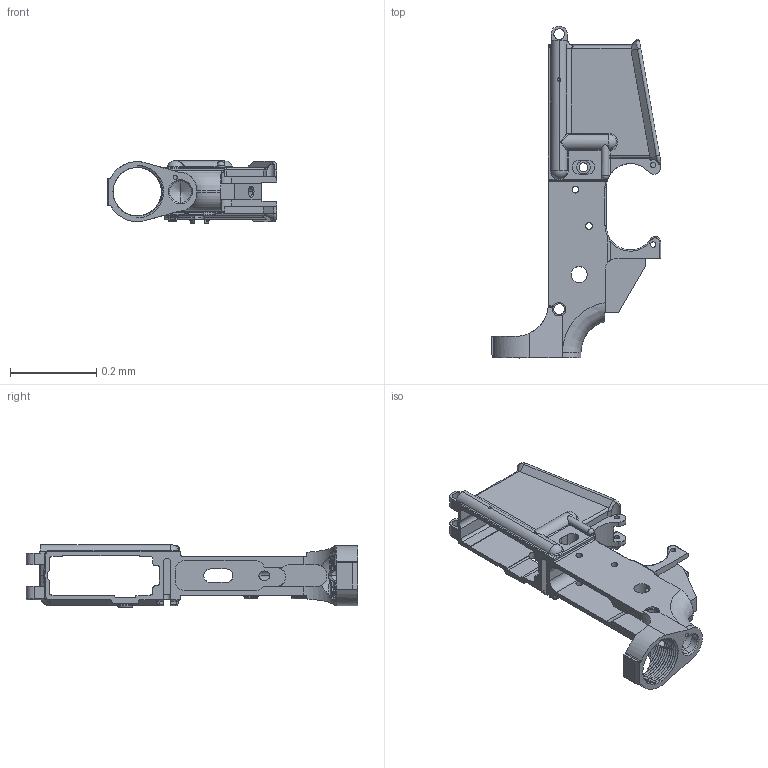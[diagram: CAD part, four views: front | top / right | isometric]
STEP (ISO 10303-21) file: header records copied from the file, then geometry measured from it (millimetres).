
FILE_DESCRIPTION(('CAx-IF Rec.Pracs.---Model Styling and Organization---1.2---2011-12-15','CAx-IF Rec.Pracs.---Geometric and Assembly Validation Properties---4.1---2014-06-16','CAx-IF Rec.Pracs.---PMI Polyline Presentation---2.0---2013-05-24'),'2;1');
FILE_NAME('AR15-lower-receiver-scale.stp','2017-10-16T01:32:52+08:00',('HyperWorksVersion-14.0.0.88'),(''),'STEP Interface 4.0 Sp3 by CT CoreTechnologie','3D_Kernel_IO4.0 Sp3 by CT CoreTechnologie','');
FILE_SCHEMA(('AUTOMOTIVE_DESIGN { 1 0 10303 214 1 1 1 1 }'));
Length unit declared in the file: millimetre
Products named in the file (1): AR15-lower-receiver-scale
Bounding box: 0.39 x 0.77 x 0.14 mm (x, y, z)
Surface area: 0.8 mm2 (no closed solid volume)
Topology: 0 solids, 2 shells, 511 faces, 1426 edges, 903 vertices
Faces by surface type: cylinder 234, plane 164, bspline 79, torus 28, sphere 6
Entity records: 40165 total; most frequent: CARTESIAN_POINT 23003, ORIENTED_EDGE 2830, DIRECTION 2675, EDGE_CURVE 1418, AXIS2_PLACEMENT_3D 976, VERTEX_POINT 906, VECTOR 723, LINE 723
